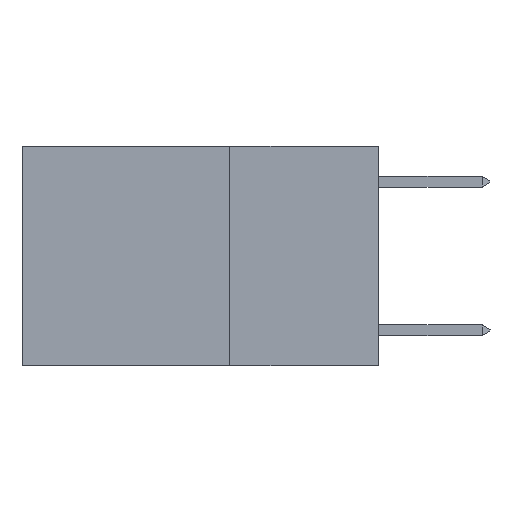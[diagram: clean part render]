
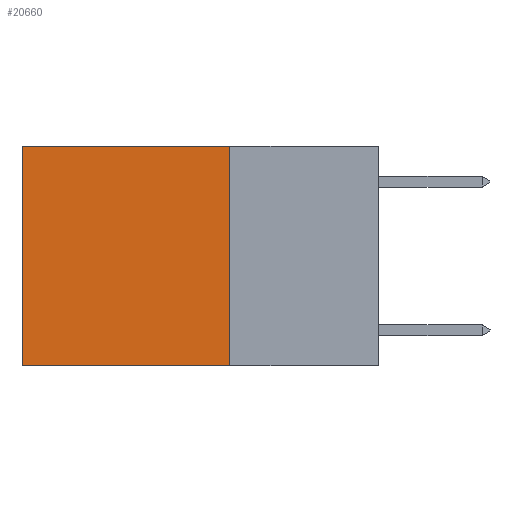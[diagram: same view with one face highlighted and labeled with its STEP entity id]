
A CAD part, left-side view. The second image highlights one B-rep face of the part: STEP entity #20660.
In plain terms, the highlighted planar face has unit normal (-1, 0, 0).
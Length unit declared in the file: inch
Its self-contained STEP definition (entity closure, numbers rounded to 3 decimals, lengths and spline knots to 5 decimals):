
#366 = ORIENTED_EDGE ( 'NONE', *, *, #7335, .F. ) ;
#392 = VERTEX_POINT ( 'NONE', #19942 ) ;
#961 = ORIENTED_EDGE ( 'NONE', *, *, #6446, .T. ) ;
#1709 = DIRECTION ( 'NONE',  ( 0., 1., 0. ) ) ;
#1835 = CARTESIAN_POINT ( 'NONE',  ( 0.2625, 0.25, -0.37 ) ) ;
#2451 = DIRECTION ( 'NONE',  ( 0., 0., -1. ) ) ;
#2586 = CARTESIAN_POINT ( 'NONE',  ( 0.2625, 0.6, 0. ) ) ;
#2656 = ORIENTED_EDGE ( 'NONE', *, *, #13299, .F. ) ;
#3999 = VERTEX_POINT ( 'NONE', #7137 ) ;
#6446 = EDGE_CURVE ( 'NONE', #3999, #392, #17042, .T. ) ;
#7137 = CARTESIAN_POINT ( 'NONE',  ( 0.2625, 0.6, 0. ) ) ;
#7335 = EDGE_CURVE ( 'NONE', #8474, #8413, #10722, .T. ) ;
#7910 = EDGE_LOOP ( 'NONE', ( #961, #2656, #366, #16430 ) ) ;
#8413 = VERTEX_POINT ( 'NONE', #17827 ) ;
#8474 = VERTEX_POINT ( 'NONE', #16678 ) ;
#9856 = VECTOR ( 'NONE', #1709, 39.37008 ) ;
#10208 = EDGE_CURVE ( 'NONE', #8474, #3999, #11451, .T. ) ;
#10593 = VECTOR ( 'NONE', #17796, 39.37008 ) ;
#10722 = LINE ( 'NONE', #17687, #10593 ) ;
#10794 = DIRECTION ( 'NONE',  ( 0., 0., -1. ) ) ;
#10797 = DIRECTION ( 'NONE',  ( 1., 0., 0. ) ) ;
#10825 = CARTESIAN_POINT ( 'NONE',  ( 0.2625, 0.25, 0. ) ) ;
#10977 = FACE_OUTER_BOUND ( 'NONE', #7910, .T. ) ;
#11016 = PLANE ( 'NONE',  #18360 ) ;
#11101 = LINE ( 'NONE', #1835, #9856 ) ;
#11400 = VECTOR ( 'NONE', #17809, 39.37008 ) ;
#11451 = LINE ( 'NONE', #17978, #11400 ) ;
#13299 = EDGE_CURVE ( 'NONE', #8413, #392, #11101, .T. ) ;
#16430 = ORIENTED_EDGE ( 'NONE', *, *, #10208, .T. ) ;
#16678 = CARTESIAN_POINT ( 'NONE',  ( 0.2625, 0.25, 0. ) ) ;
#16879 = VECTOR ( 'NONE', #2451, 39.37008 ) ;
#17042 = LINE ( 'NONE', #2586, #16879 ) ;
#17687 = CARTESIAN_POINT ( 'NONE',  ( 0.2625, 0.25, 0. ) ) ;
#17796 = DIRECTION ( 'NONE',  ( 0., 0., -1. ) ) ;
#17809 = DIRECTION ( 'NONE',  ( 0., 1., 0. ) ) ;
#17827 = CARTESIAN_POINT ( 'NONE',  ( 0.2625, 0.25, -0.37 ) ) ;
#17978 = CARTESIAN_POINT ( 'NONE',  ( 0.2625, 0.25, 0. ) ) ;
#18360 = AXIS2_PLACEMENT_3D ( 'NONE', #10825, #10797, #10794 ) ;
#19942 = CARTESIAN_POINT ( 'NONE',  ( 0.2625, 0.6, -0.37 ) ) ;
#20660 = ADVANCED_FACE ( 'NONE', ( #10977 ), #11016, .F. ) ;
